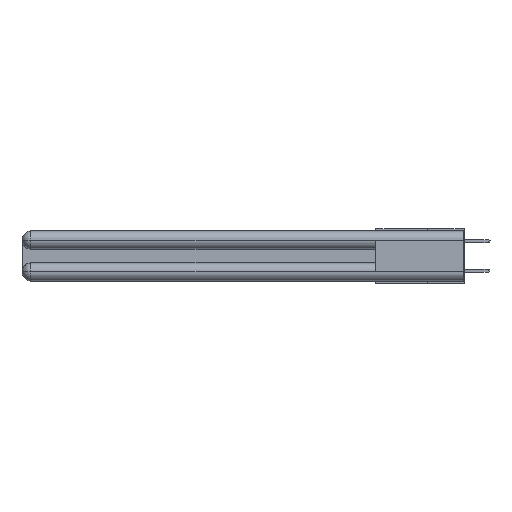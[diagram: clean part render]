
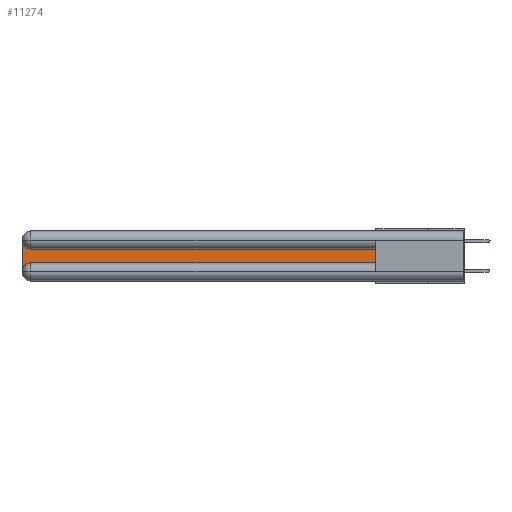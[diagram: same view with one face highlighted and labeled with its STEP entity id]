
A CAD part, left-side view. The second image highlights one B-rep face of the part: STEP entity #11274.
In plain terms, the highlighted planar face has unit normal (-1, 0, 0).
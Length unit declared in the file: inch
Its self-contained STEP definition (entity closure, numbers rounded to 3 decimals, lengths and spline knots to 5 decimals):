
#325 = CIRCLE ( 'NONE', #28314, 0.06 ) ;
#1895 = CARTESIAN_POINT ( 'NONE',  ( 0.075, 2.94, -0.0625 ) ) ;
#2262 = LINE ( 'NONE', #13604, #11025 ) ;
#2519 = DIRECTION ( 'NONE',  ( 1., 0., 0. ) ) ;
#2779 = VERTEX_POINT ( 'NONE', #18325 ) ;
#2821 = DIRECTION ( 'NONE',  ( 0., 0., -1. ) ) ;
#3268 = LINE ( 'NONE', #25272, #21832 ) ;
#3555 = VECTOR ( 'NONE', #19950, 39.37008 ) ;
#4653 = ORIENTED_EDGE ( 'NONE', *, *, #16209, .T. ) ;
#5371 = CARTESIAN_POINT ( 'NONE',  ( 0.075, 2.94, -0.2775 ) ) ;
#6598 = VERTEX_POINT ( 'NONE', #20129 ) ;
#6856 = ORIENTED_EDGE ( 'NONE', *, *, #28527, .T. ) ;
#8179 = CIRCLE ( 'NONE', #29530, 0.06 ) ;
#8779 = VECTOR ( 'NONE', #28603, 39.37008 ) ;
#8992 = EDGE_CURVE ( 'NONE', #6598, #2779, #10124, .T. ) ;
#9297 = CARTESIAN_POINT ( 'NONE',  ( 0.075, 2.94, -0.1225 ) ) ;
#10062 = DIRECTION ( 'NONE',  ( 1., 0., 0. ) ) ;
#10124 = LINE ( 'NONE', #25660, #3555 ) ;
#11005 = EDGE_CURVE ( 'NONE', #2779, #21425, #325, .T. ) ;
#11025 = VECTOR ( 'NONE', #20605, 39.37008 ) ;
#11045 = ORIENTED_EDGE ( 'NONE', *, *, #26143, .T. ) ;
#11163 = CARTESIAN_POINT ( 'NONE',  ( 0.075, 0.6, -0.1225 ) ) ;
#11239 = CARTESIAN_POINT ( 'NONE',  ( 0.075, 0.6, -0.2175 ) ) ;
#11274 = ADVANCED_FACE ( 'NONE', ( #27239 ), #16259, .F. ) ;
#11857 = CARTESIAN_POINT ( 'NONE',  ( 0.075, 0.6, -0.1225 ) ) ;
#13604 = CARTESIAN_POINT ( 'NONE',  ( 0.075, 0.6, -0.2175 ) ) ;
#15195 = EDGE_CURVE ( 'NONE', #20042, #16004, #2262, .T. ) ;
#16004 = VERTEX_POINT ( 'NONE', #11163 ) ;
#16209 = EDGE_CURVE ( 'NONE', #16004, #27254, #27311, .T. ) ;
#16259 = PLANE ( 'NONE',  #17221 ) ;
#17221 = AXIS2_PLACEMENT_3D ( 'NONE', #23270, #2519, #2821 ) ;
#18077 = DIRECTION ( 'NONE',  ( 0., 0., -1. ) ) ;
#18302 = ORIENTED_EDGE ( 'NONE', *, *, #8992, .T. ) ;
#18325 = CARTESIAN_POINT ( 'NONE',  ( 0.075, 3., -0.2775 ) ) ;
#19950 = DIRECTION ( 'NONE',  ( 0., 0., -1. ) ) ;
#20042 = VERTEX_POINT ( 'NONE', #11239 ) ;
#20129 = CARTESIAN_POINT ( 'NONE',  ( 0.075, 3., -0.0625 ) ) ;
#20605 = DIRECTION ( 'NONE',  ( 0., 0., 1. ) ) ;
#21425 = VERTEX_POINT ( 'NONE', #22529 ) ;
#21608 = DIRECTION ( 'NONE',  ( 0., 0., -1. ) ) ;
#21832 = VECTOR ( 'NONE', #25890, 39.37008 ) ;
#22233 = ORIENTED_EDGE ( 'NONE', *, *, #11005, .T. ) ;
#22529 = CARTESIAN_POINT ( 'NONE',  ( 0.075, 2.94, -0.2175 ) ) ;
#23270 = CARTESIAN_POINT ( 'NONE',  ( 0.075, 3., -0.1225 ) ) ;
#24495 = ORIENTED_EDGE ( 'NONE', *, *, #15195, .T. ) ;
#24884 = DIRECTION ( 'NONE',  ( 1., 0., 0. ) ) ;
#25272 = CARTESIAN_POINT ( 'NONE',  ( 0.075, 0.6, -0.2175 ) ) ;
#25660 = CARTESIAN_POINT ( 'NONE',  ( 0.075, 3., -0.2175 ) ) ;
#25890 = DIRECTION ( 'NONE',  ( 0., -1., 0. ) ) ;
#26143 = EDGE_CURVE ( 'NONE', #27254, #6598, #8179, .T. ) ;
#26416 = EDGE_LOOP ( 'NONE', ( #4653, #11045, #18302, #22233, #6856, #24495 ) ) ;
#27239 = FACE_OUTER_BOUND ( 'NONE', #26416, .T. ) ;
#27254 = VERTEX_POINT ( 'NONE', #9297 ) ;
#27311 = LINE ( 'NONE', #11857, #8779 ) ;
#28314 = AXIS2_PLACEMENT_3D ( 'NONE', #5371, #10062, #21608 ) ;
#28527 = EDGE_CURVE ( 'NONE', #21425, #20042, #3268, .T. ) ;
#28603 = DIRECTION ( 'NONE',  ( 0., 1., 0. ) ) ;
#29530 = AXIS2_PLACEMENT_3D ( 'NONE', #1895, #24884, #18077 ) ;
